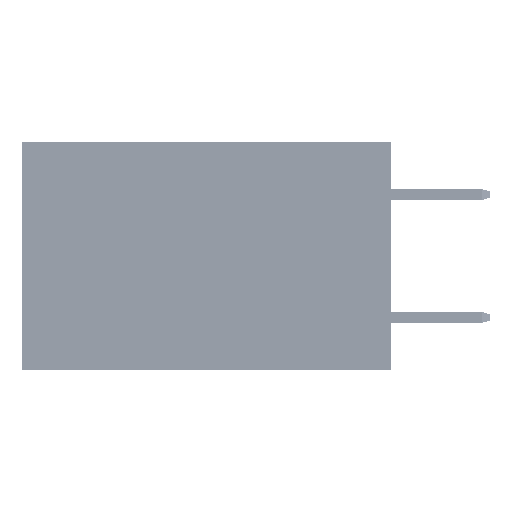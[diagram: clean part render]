
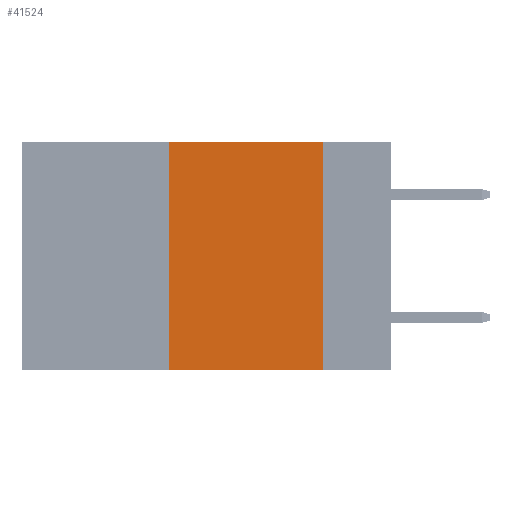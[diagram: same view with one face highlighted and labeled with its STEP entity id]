
A CAD part, left-side view. The second image highlights one B-rep face of the part: STEP entity #41524.
In plain terms, the highlighted planar face has unit normal (-1, 0, 0).
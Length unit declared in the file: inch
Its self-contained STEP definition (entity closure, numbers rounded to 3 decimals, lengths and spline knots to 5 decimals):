
#1662 = VECTOR ( 'NONE', #38809, 39.37008 ) ;
#2366 = ORIENTED_EDGE ( 'NONE', *, *, #12232, .T. ) ;
#2472 = DIRECTION ( 'NONE',  ( 0., 0., -1. ) ) ;
#3131 = DIRECTION ( 'NONE',  ( 0., 0., -1. ) ) ;
#4448 = VERTEX_POINT ( 'NONE', #33784 ) ;
#4504 = DIRECTION ( 'NONE',  ( 0., -1., 0. ) ) ;
#5374 = EDGE_LOOP ( 'NONE', ( #34769, #32113, #37488, #2366 ) ) ;
#5540 = EDGE_CURVE ( 'NONE', #42613, #5542, #28805, .T. ) ;
#5542 = VERTEX_POINT ( 'NONE', #17139 ) ;
#12232 = EDGE_CURVE ( 'NONE', #4448, #5542, #16641, .T. ) ;
#12952 = PLANE ( 'NONE',  #24205 ) ;
#13119 = CARTESIAN_POINT ( 'NONE',  ( 0., 0.36, 0. ) ) ;
#13425 = CARTESIAN_POINT ( 'NONE',  ( 0., 0.6, -0.37 ) ) ;
#15258 = CARTESIAN_POINT ( 'NONE',  ( 0., 0.6, 0. ) ) ;
#16641 = LINE ( 'NONE', #13425, #40173 ) ;
#17139 = CARTESIAN_POINT ( 'NONE',  ( 0., 0.11, -0.37 ) ) ;
#20789 = DIRECTION ( 'NONE',  ( 0., -1., 0. ) ) ;
#24205 = AXIS2_PLACEMENT_3D ( 'NONE', #46249, #46410, #2472 ) ;
#28228 = VECTOR ( 'NONE', #4504, 39.37008 ) ;
#28805 = LINE ( 'NONE', #36241, #42023 ) ;
#29353 = LINE ( 'NONE', #15258, #28228 ) ;
#32113 = ORIENTED_EDGE ( 'NONE', *, *, #34889, .F. ) ;
#33784 = CARTESIAN_POINT ( 'NONE',  ( 0., 0.36, -0.37 ) ) ;
#34769 = ORIENTED_EDGE ( 'NONE', *, *, #5540, .F. ) ;
#34889 = EDGE_CURVE ( 'NONE', #43231, #42613, #29353, .T. ) ;
#35224 = FACE_OUTER_BOUND ( 'NONE', #5374, .T. ) ;
#35607 = CARTESIAN_POINT ( 'NONE',  ( 0., 0.11, 0. ) ) ;
#35612 = LINE ( 'NONE', #13119, #1662 ) ;
#35755 = EDGE_CURVE ( 'NONE', #4448, #43231, #35612, .T. ) ;
#36241 = CARTESIAN_POINT ( 'NONE',  ( 0., 0.11, 0. ) ) ;
#37488 = ORIENTED_EDGE ( 'NONE', *, *, #35755, .F. ) ;
#38759 = CARTESIAN_POINT ( 'NONE',  ( 0., 0.36, 0. ) ) ;
#38809 = DIRECTION ( 'NONE',  ( 0., 0., 1. ) ) ;
#40173 = VECTOR ( 'NONE', #20789, 39.37008 ) ;
#41524 = ADVANCED_FACE ( 'NONE', ( #35224 ), #12952, .F. ) ;
#42023 = VECTOR ( 'NONE', #3131, 39.37008 ) ;
#42613 = VERTEX_POINT ( 'NONE', #35607 ) ;
#43231 = VERTEX_POINT ( 'NONE', #38759 ) ;
#46249 = CARTESIAN_POINT ( 'NONE',  ( 0., 0.6, 0. ) ) ;
#46410 = DIRECTION ( 'NONE',  ( 1., 0., 0. ) ) ;
